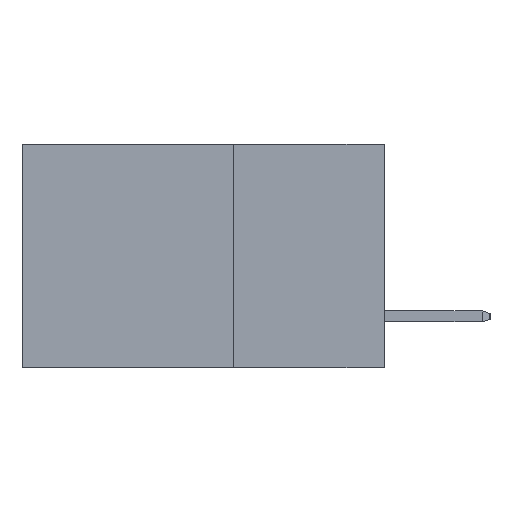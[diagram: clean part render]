
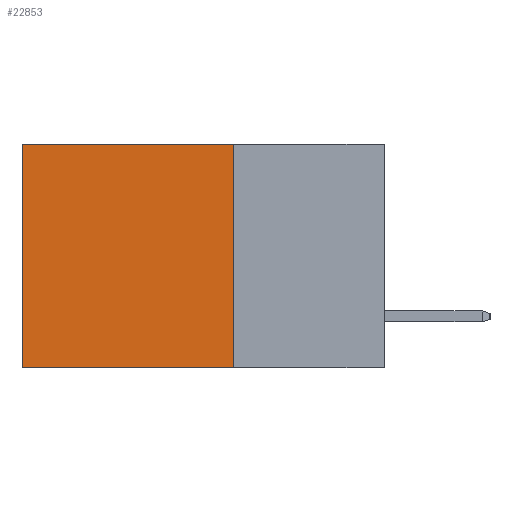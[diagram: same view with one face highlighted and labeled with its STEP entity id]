
A CAD part, left-side view. The second image highlights one B-rep face of the part: STEP entity #22853.
In plain terms, the highlighted planar face has unit normal (-1, 0, 0).
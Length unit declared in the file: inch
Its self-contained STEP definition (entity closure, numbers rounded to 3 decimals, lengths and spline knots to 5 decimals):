
#1164 = CARTESIAN_POINT ( 'NONE',  ( 0.2615, 0.6, 0. ) ) ;
#1516 = DIRECTION ( 'NONE',  ( 0., 0., -1. ) ) ;
#1671 = VECTOR ( 'NONE', #1516, 39.37008 ) ;
#2210 = CARTESIAN_POINT ( 'NONE',  ( 0.2615, 0.6, -0.37 ) ) ;
#2441 = VECTOR ( 'NONE', #17437, 39.37008 ) ;
#3743 = EDGE_CURVE ( 'NONE', #11460, #21458, #16793, .T. ) ;
#4378 = LINE ( 'NONE', #8470, #22565 ) ;
#5921 = EDGE_LOOP ( 'NONE', ( #6936, #19060, #12283, #16851 ) ) ;
#6574 = VERTEX_POINT ( 'NONE', #12062 ) ;
#6645 = CARTESIAN_POINT ( 'NONE',  ( 0.2615, 0.25, -0.37 ) ) ;
#6647 = DIRECTION ( 'NONE',  ( 0., 1., 0. ) ) ;
#6724 = CARTESIAN_POINT ( 'NONE',  ( 0.2615, 0.25, 0. ) ) ;
#6936 = ORIENTED_EDGE ( 'NONE', *, *, #3743, .T. ) ;
#8100 = DIRECTION ( 'NONE',  ( 0., 1., 0. ) ) ;
#8470 = CARTESIAN_POINT ( 'NONE',  ( 0.2615, 0.25, -0.37 ) ) ;
#8503 = DIRECTION ( 'NONE',  ( 1., 0., 0. ) ) ;
#9703 = AXIS2_PLACEMENT_3D ( 'NONE', #6645, #8503, #20857 ) ;
#10244 = PLANE ( 'NONE',  #9703 ) ;
#10403 = EDGE_CURVE ( 'NONE', #15006, #21458, #4378, .T. ) ;
#11284 = LINE ( 'NONE', #22802, #1671 ) ;
#11326 = VECTOR ( 'NONE', #6647, 39.37008 ) ;
#11460 = VERTEX_POINT ( 'NONE', #1164 ) ;
#12062 = CARTESIAN_POINT ( 'NONE',  ( 0.2615, 0.25, 0. ) ) ;
#12283 = ORIENTED_EDGE ( 'NONE', *, *, #21237, .F. ) ;
#12838 = EDGE_CURVE ( 'NONE', #6574, #11460, #17187, .T. ) ;
#14146 = CARTESIAN_POINT ( 'NONE',  ( 0.2615, 0.6, -0.37 ) ) ;
#15006 = VERTEX_POINT ( 'NONE', #16483 ) ;
#16483 = CARTESIAN_POINT ( 'NONE',  ( 0.2615, 0.25, -0.37 ) ) ;
#16793 = LINE ( 'NONE', #14146, #2441 ) ;
#16851 = ORIENTED_EDGE ( 'NONE', *, *, #12838, .T. ) ;
#17187 = LINE ( 'NONE', #6724, #11326 ) ;
#17437 = DIRECTION ( 'NONE',  ( 0., 0., -1. ) ) ;
#17728 = FACE_OUTER_BOUND ( 'NONE', #5921, .T. ) ;
#19060 = ORIENTED_EDGE ( 'NONE', *, *, #10403, .F. ) ;
#20857 = DIRECTION ( 'NONE',  ( 0., 0., -1. ) ) ;
#21237 = EDGE_CURVE ( 'NONE', #6574, #15006, #11284, .T. ) ;
#21458 = VERTEX_POINT ( 'NONE', #2210 ) ;
#22565 = VECTOR ( 'NONE', #8100, 39.37008 ) ;
#22802 = CARTESIAN_POINT ( 'NONE',  ( 0.2615, 0.25, -0.37 ) ) ;
#22853 = ADVANCED_FACE ( 'NONE', ( #17728 ), #10244, .F. ) ;
